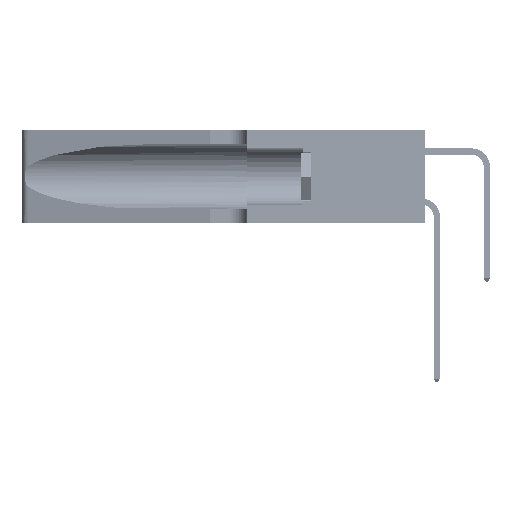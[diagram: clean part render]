
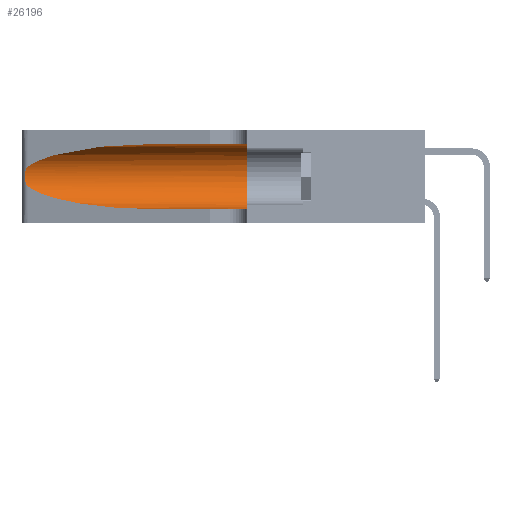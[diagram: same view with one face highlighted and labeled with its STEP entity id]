
A CAD part, left-side view. The second image highlights one B-rep face of the part: STEP entity #26196.
In plain terms, the highlighted cylindrical face has radius 3.308 mm (diameter 6.617 mm), a partial arc.
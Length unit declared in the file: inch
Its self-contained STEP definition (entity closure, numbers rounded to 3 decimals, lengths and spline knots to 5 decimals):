
#70 = CARTESIAN_POINT ( 'NONE',  ( 0.25639, 1.23186, 0.15144 ) ) ;
#1788 = CARTESIAN_POINT ( 'NONE',  ( 0.25487, 1.22718, 0.14631 ) ) ;
#2918 = CARTESIAN_POINT ( 'NONE',  ( 0.1305, 0.35, 0.185 ) ) ;
#5875 = CARTESIAN_POINT ( 'NONE',  ( 0.1305, 0.72297, 0.31525 ) ) ;
#6309 = EDGE_CURVE ( 'NONE', #14005, #36362, #47704, .T. ) ;
#7197 = VERTEX_POINT ( 'NONE', #39706 ) ;
#7624 = VECTOR ( 'NONE', #39971, 39.37008 ) ;
#7950 = CARTESIAN_POINT ( 'NONE',  ( 0.25555, 1.22994, 0.2215 ) ) ;
#8211 = LINE ( 'NONE', #20378, #7624 ) ;
#8542 = CARTESIAN_POINT ( 'NONE',  ( 0.1305, 0.35, 0.05475 ) ) ;
#10270 = CARTESIAN_POINT ( 'NONE',  ( 0.1305, 0.35, 0.31525 ) ) ;
#10562 = CARTESIAN_POINT ( 'NONE',  ( 0.25487, 1.22718, 0.22369 ) ) ;
#11016 = CARTESIAN_POINT ( 'NONE',  ( 0.1305, 0.72297, 0.05475 ) ) ;
#11614 = LINE ( 'NONE', #38150, #22899 ) ;
#11950 = CARTESIAN_POINT ( 'NONE',  ( 0.25854, 1.2359, 0.20912 ) ) ;
#12231 = CARTESIAN_POINT ( 'NONE',  ( 0.25487, 1.22718, 0.14631 ) ) ;
#12481 = CARTESIAN_POINT ( 'NONE',  ( 0.26075, 1.23896, 0.19203 ) ) ;
#13861 = ORIENTED_EDGE ( 'NONE', *, *, #36771, .T. ) ;
#14005 = VERTEX_POINT ( 'NONE', #12231 ) ;
#16347 = CARTESIAN_POINT ( 'NONE',  ( 0.26075, 1.23896, 0.178 ) ) ;
#16715 = CARTESIAN_POINT ( 'NONE',  ( 0.26018, 1.23835, 0.19895 ) ) ;
#18271 = CARTESIAN_POINT ( 'NONE',  ( 0.2373, 1.15595, 0.08982 ) ) ;
#18756 =( BOUNDED_CURVE ( )  B_SPLINE_CURVE ( 3, ( #34391, #38240, #30208, #10562 ),
 .UNSPECIFIED., .F., .T. ) 
 B_SPLINE_CURVE_WITH_KNOTS ( ( 4, 4 ),
 ( 1.5708, 2.84003 ),
 .UNSPECIFIED. ) 
 CURVE ( )  GEOMETRIC_REPRESENTATION_ITEM ( )  RATIONAL_B_SPLINE_CURVE ( ( 1., 0.87, 0.87, 1. ) ) 
 REPRESENTATION_ITEM ( '' )  );
#18887 = EDGE_CURVE ( 'NONE', #36362, #22279, #11614, .T. ) ;
#20030 = DIRECTION ( 'NONE',  ( 0., -1., 0. ) ) ;
#20049 = CARTESIAN_POINT ( 'NONE',  ( 0.25787, 1.23484, 0.2124 ) ) ;
#20378 = CARTESIAN_POINT ( 'NONE',  ( 0.1305, 1.61858, 0.31525 ) ) ;
#20466 = ORIENTED_EDGE ( 'NONE', *, *, #46339, .T. ) ;
#21898 = ORIENTED_EDGE ( 'NONE', *, *, #41603, .F. ) ;
#22279 = VERTEX_POINT ( 'NONE', #8542 ) ;
#22514 = VERTEX_POINT ( 'NONE', #10270 ) ;
#22899 = VECTOR ( 'NONE', #34298, 39.37008 ) ;
#23439 = DIRECTION ( 'NONE',  ( 0., 1., 0. ) ) ;
#24076 = CARTESIAN_POINT ( 'NONE',  ( 0.25789, 1.23486, 0.15765 ) ) ;
#24614 = CARTESIAN_POINT ( 'NONE',  ( 0.25639, 1.23184, 0.21858 ) ) ;
#24727 = CIRCLE ( 'NONE', #47531, 0.13025 ) ;
#25758 = VERTEX_POINT ( 'NONE', #5875 ) ;
#26196 = ADVANCED_FACE ( 'NONE', ( #36320 ), #41368, .F. ) ;
#27474 = DIRECTION ( 'NONE',  ( 0., 0., 1. ) ) ;
#28111 = CARTESIAN_POINT ( 'NONE',  ( 0.25555, 1.22993, 0.14849 ) ) ;
#28300 = EDGE_LOOP ( 'NONE', ( #13861, #20466, #45373, #43907, #21898, #33433 ) ) ;
#29662 = CARTESIAN_POINT ( 'NONE',  ( 0.18966, 0.96281, 0.05475 ) ) ;
#30208 = CARTESIAN_POINT ( 'NONE',  ( 0.2373, 1.15595, 0.28018 ) ) ;
#33433 = ORIENTED_EDGE ( 'NONE', *, *, #43034, .F. ) ;
#33689 = CARTESIAN_POINT ( 'NONE',  ( 0.1305, 0.72297, 0.05475 ) ) ;
#34298 = DIRECTION ( 'NONE',  ( 0., -1., 0. ) ) ;
#34391 = CARTESIAN_POINT ( 'NONE',  ( 0.1305, 0.72297, 0.31525 ) ) ;
#36276 = DIRECTION ( 'NONE',  ( 0., 0., -1. ) ) ;
#36320 = FACE_OUTER_BOUND ( 'NONE', #28300, .T. ) ;
#36362 = VERTEX_POINT ( 'NONE', #11016 ) ;
#36486 = CARTESIAN_POINT ( 'NONE',  ( 0.26017, 1.23833, 0.17102 ) ) ;
#36771 = EDGE_CURVE ( 'NONE', #25758, #7197, #18756, .T. ) ;
#38150 = CARTESIAN_POINT ( 'NONE',  ( 0.1305, 1.61858, 0.05475 ) ) ;
#38240 = CARTESIAN_POINT ( 'NONE',  ( 0.18966, 0.96281, 0.31525 ) ) ;
#39706 = CARTESIAN_POINT ( 'NONE',  ( 0.25487, 1.22718, 0.22369 ) ) ;
#39971 = DIRECTION ( 'NONE',  ( 0., -1., 0. ) ) ;
#40335 = CARTESIAN_POINT ( 'NONE',  ( 0.25487, 1.22718, 0.14631 ) ) ;
#41368 = CYLINDRICAL_SURFACE ( 'NONE', #48167, 0.13025 ) ;
#41603 = EDGE_CURVE ( 'NONE', #22514, #22279, #24727, .T. ) ;
#43034 = EDGE_CURVE ( 'NONE', #25758, #22514, #8211, .T. ) ;
#43907 = ORIENTED_EDGE ( 'NONE', *, *, #18887, .T. ) ;
#44175 = CARTESIAN_POINT ( 'NONE',  ( 0.25487, 1.22718, 0.22369 ) ) ;
#44719 = CARTESIAN_POINT ( 'NONE',  ( 0.25856, 1.23593, 0.16098 ) ) ;
#45373 = ORIENTED_EDGE ( 'NONE', *, *, #6309, .T. ) ;
#46339 = EDGE_CURVE ( 'NONE', #7197, #14005, #51435, .T. ) ;
#47531 = AXIS2_PLACEMENT_3D ( 'NONE', #2918, #23439, #27474 ) ;
#47704 =( BOUNDED_CURVE ( )  B_SPLINE_CURVE ( 3, ( #1788, #18271, #29662, #33689 ),
 .UNSPECIFIED., .F., .F. ) 
 B_SPLINE_CURVE_WITH_KNOTS ( ( 4, 4 ),
 ( 3.44316, 4.71239 ),
 .UNSPECIFIED. ) 
 CURVE ( )  GEOMETRIC_REPRESENTATION_ITEM ( )  RATIONAL_B_SPLINE_CURVE ( ( 1., 0.87, 0.87, 1. ) ) 
 REPRESENTATION_ITEM ( '' )  );
#48167 = AXIS2_PLACEMENT_3D ( 'NONE', #51707, #20030, #36276 ) ;
#51435 = B_SPLINE_CURVE_WITH_KNOTS ( 'NONE', 3,
 ( #44175, #7950, #24614, #20049, #11950, #16715, #12481, #16347, #36486, #44719, #24076, #70, #28111, #40335 ),
 .UNSPECIFIED., .F., .F.,
 ( 4, 2, 2, 2, 2, 2, 4 ),
 ( 0., 0.00027, 0.00053, 0.00107, 0.0016, 0.00187, 0.00214 ),
 .UNSPECIFIED. ) ;
#51707 = CARTESIAN_POINT ( 'NONE',  ( 0.1305, 1.61858, 0.185 ) ) ;
